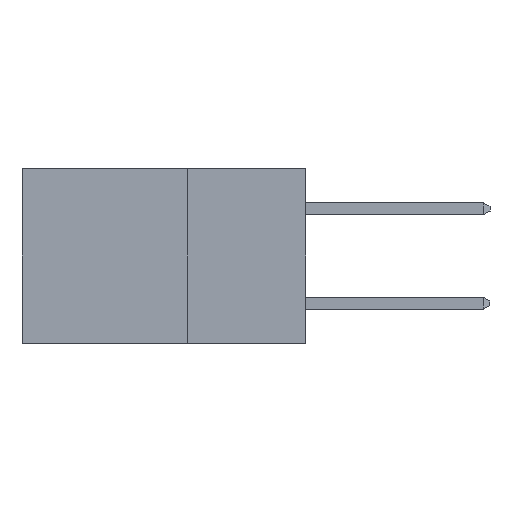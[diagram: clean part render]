
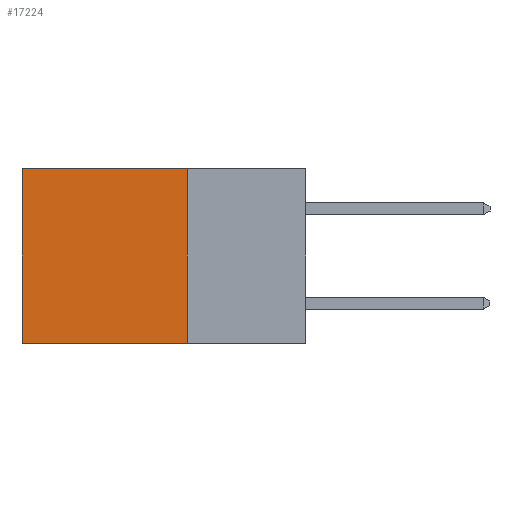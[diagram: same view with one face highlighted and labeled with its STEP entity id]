
A CAD part, left-side view. The second image highlights one B-rep face of the part: STEP entity #17224.
In plain terms, the highlighted planar face has unit normal (-1, 0, 0).
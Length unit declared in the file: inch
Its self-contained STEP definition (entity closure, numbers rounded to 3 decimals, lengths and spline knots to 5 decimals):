
#140 = DIRECTION ( 'NONE',  ( 0., 1., 0. ) ) ;
#607 = CARTESIAN_POINT ( 'NONE',  ( 0.298, 0.25, -0.37 ) ) ;
#753 = VECTOR ( 'NONE', #6283, 39.37008 ) ;
#1202 = AXIS2_PLACEMENT_3D ( 'NONE', #14635, #21794, #11049 ) ;
#1848 = ORIENTED_EDGE ( 'NONE', *, *, #18702, .F. ) ;
#1884 = LINE ( 'NONE', #13058, #15933 ) ;
#2755 = FACE_OUTER_BOUND ( 'NONE', #4643, .T. ) ;
#4643 = EDGE_LOOP ( 'NONE', ( #4750, #16939, #1848, #11853 ) ) ;
#4750 = ORIENTED_EDGE ( 'NONE', *, *, #7727, .T. ) ;
#6276 = CARTESIAN_POINT ( 'NONE',  ( 0.298, 0.6, 0. ) ) ;
#6283 = DIRECTION ( 'NONE',  ( 0., 0., -1. ) ) ;
#7727 = EDGE_CURVE ( 'NONE', #10099, #10236, #15969, .T. ) ;
#7981 = VERTEX_POINT ( 'NONE', #607 ) ;
#8874 = VECTOR ( 'NONE', #11000, 39.37008 ) ;
#9198 = PLANE ( 'NONE',  #1202 ) ;
#10099 = VERTEX_POINT ( 'NONE', #15625 ) ;
#10236 = VERTEX_POINT ( 'NONE', #23105 ) ;
#10502 = VECTOR ( 'NONE', #14328, 39.37008 ) ;
#11000 = DIRECTION ( 'NONE',  ( 0., 1., 0. ) ) ;
#11049 = DIRECTION ( 'NONE',  ( 0., 0., -1. ) ) ;
#11193 = VERTEX_POINT ( 'NONE', #19401 ) ;
#11853 = ORIENTED_EDGE ( 'NONE', *, *, #12852, .T. ) ;
#12852 = EDGE_CURVE ( 'NONE', #11193, #10099, #1884, .T. ) ;
#13058 = CARTESIAN_POINT ( 'NONE',  ( 0.298, 0.25, 0. ) ) ;
#14328 = DIRECTION ( 'NONE',  ( 0., 0., -1. ) ) ;
#14635 = CARTESIAN_POINT ( 'NONE',  ( 0.298, 0.25, 0. ) ) ;
#15337 = LINE ( 'NONE', #19656, #10502 ) ;
#15625 = CARTESIAN_POINT ( 'NONE',  ( 0.298, 0.6, 0. ) ) ;
#15933 = VECTOR ( 'NONE', #140, 39.37008 ) ;
#15969 = LINE ( 'NONE', #6276, #753 ) ;
#16939 = ORIENTED_EDGE ( 'NONE', *, *, #22688, .F. ) ;
#17224 = ADVANCED_FACE ( 'NONE', ( #2755 ), #9198, .F. ) ;
#18702 = EDGE_CURVE ( 'NONE', #11193, #7981, #15337, .T. ) ;
#19401 = CARTESIAN_POINT ( 'NONE',  ( 0.298, 0.25, 0. ) ) ;
#19656 = CARTESIAN_POINT ( 'NONE',  ( 0.298, 0.25, 0. ) ) ;
#21740 = CARTESIAN_POINT ( 'NONE',  ( 0.298, 0.25, -0.37 ) ) ;
#21794 = DIRECTION ( 'NONE',  ( 1., 0., 0. ) ) ;
#22125 = LINE ( 'NONE', #21740, #8874 ) ;
#22688 = EDGE_CURVE ( 'NONE', #7981, #10236, #22125, .T. ) ;
#23105 = CARTESIAN_POINT ( 'NONE',  ( 0.298, 0.6, -0.37 ) ) ;
